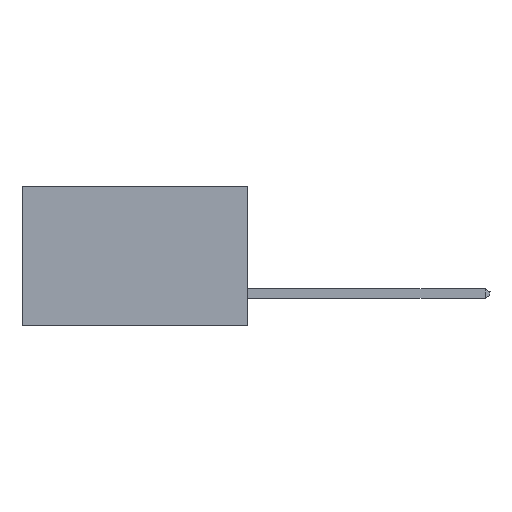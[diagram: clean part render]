
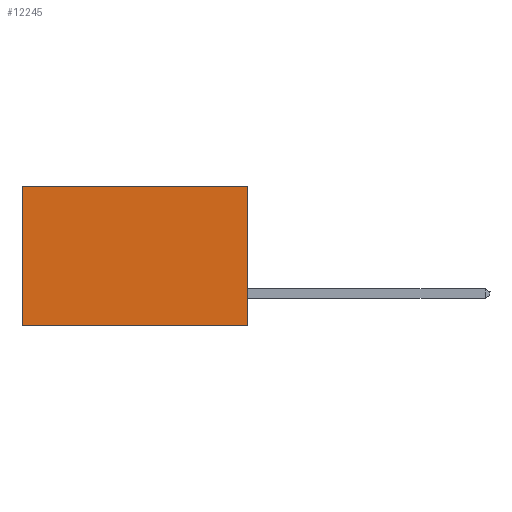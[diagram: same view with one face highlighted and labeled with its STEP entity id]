
A CAD part, left-side view. The second image highlights one B-rep face of the part: STEP entity #12245.
In plain terms, the highlighted planar face has unit normal (-1, 0, 0).
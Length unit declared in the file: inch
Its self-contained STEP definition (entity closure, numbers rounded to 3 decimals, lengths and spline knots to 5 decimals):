
#25 = AXIS2_PLACEMENT_3D ( 'NONE', #15263, #2924, #4433 ) ;
#359 = CARTESIAN_POINT ( 'NONE',  ( 0.2615, 0.6, -0.37 ) ) ;
#376 = VECTOR ( 'NONE', #9146, 39.37008 ) ;
#988 = LINE ( 'NONE', #6192, #6950 ) ;
#1792 = ORIENTED_EDGE ( 'NONE', *, *, #8132, .T. ) ;
#2080 = CARTESIAN_POINT ( 'NONE',  ( 0.2615, 0., -0.37 ) ) ;
#2924 = DIRECTION ( 'NONE',  ( 1., 0., 0. ) ) ;
#2929 = CARTESIAN_POINT ( 'NONE',  ( 0.2615, 0., 0. ) ) ;
#4177 = VERTEX_POINT ( 'NONE', #359 ) ;
#4433 = DIRECTION ( 'NONE',  ( 0., 0., -1. ) ) ;
#4497 = VERTEX_POINT ( 'NONE', #5117 ) ;
#5117 = CARTESIAN_POINT ( 'NONE',  ( 0.2615, 0., -0.37 ) ) ;
#6192 = CARTESIAN_POINT ( 'NONE',  ( 0.2615, 0., 0. ) ) ;
#6746 = ORIENTED_EDGE ( 'NONE', *, *, #9519, .F. ) ;
#6815 = CARTESIAN_POINT ( 'NONE',  ( 0.2615, 0., -0.37 ) ) ;
#6950 = VECTOR ( 'NONE', #18559, 39.37008 ) ;
#7186 = VERTEX_POINT ( 'NONE', #18400 ) ;
#8132 = EDGE_CURVE ( 'NONE', #7186, #4177, #14947, .T. ) ;
#8137 = PLANE ( 'NONE',  #25 ) ;
#8159 = EDGE_CURVE ( 'NONE', #11308, #7186, #988, .T. ) ;
#8541 = LINE ( 'NONE', #6815, #13485 ) ;
#9146 = DIRECTION ( 'NONE',  ( 0., 0., -1. ) ) ;
#9519 = EDGE_CURVE ( 'NONE', #4497, #4177, #8541, .T. ) ;
#11308 = VERTEX_POINT ( 'NONE', #2929 ) ;
#11438 = DIRECTION ( 'NONE',  ( 0., 0., -1. ) ) ;
#12245 = ADVANCED_FACE ( 'NONE', ( #15143 ), #8137, .F. ) ;
#13485 = VECTOR ( 'NONE', #21036, 39.37008 ) ;
#14947 = LINE ( 'NONE', #20425, #18534 ) ;
#15143 = FACE_OUTER_BOUND ( 'NONE', #21131, .T. ) ;
#15263 = CARTESIAN_POINT ( 'NONE',  ( 0.2615, 0., -0.37 ) ) ;
#17160 = ORIENTED_EDGE ( 'NONE', *, *, #19454, .F. ) ;
#17932 = LINE ( 'NONE', #2080, #376 ) ;
#18400 = CARTESIAN_POINT ( 'NONE',  ( 0.2615, 0.6, 0. ) ) ;
#18534 = VECTOR ( 'NONE', #11438, 39.37008 ) ;
#18559 = DIRECTION ( 'NONE',  ( 0., 1., 0. ) ) ;
#19454 = EDGE_CURVE ( 'NONE', #11308, #4497, #17932, .T. ) ;
#20425 = CARTESIAN_POINT ( 'NONE',  ( 0.2615, 0.6, -0.37 ) ) ;
#20911 = ORIENTED_EDGE ( 'NONE', *, *, #8159, .T. ) ;
#21036 = DIRECTION ( 'NONE',  ( 0., 1., 0. ) ) ;
#21131 = EDGE_LOOP ( 'NONE', ( #1792, #6746, #17160, #20911 ) ) ;
